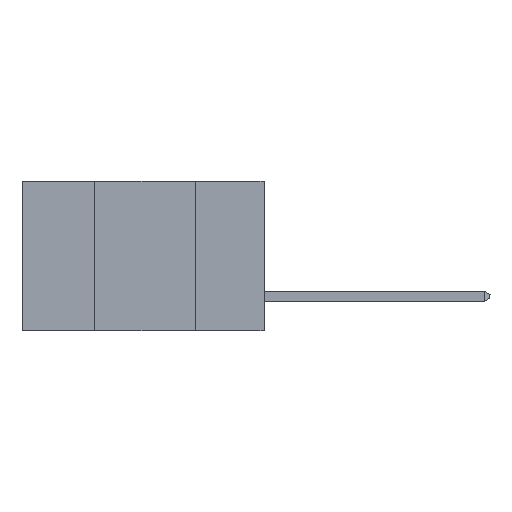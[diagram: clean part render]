
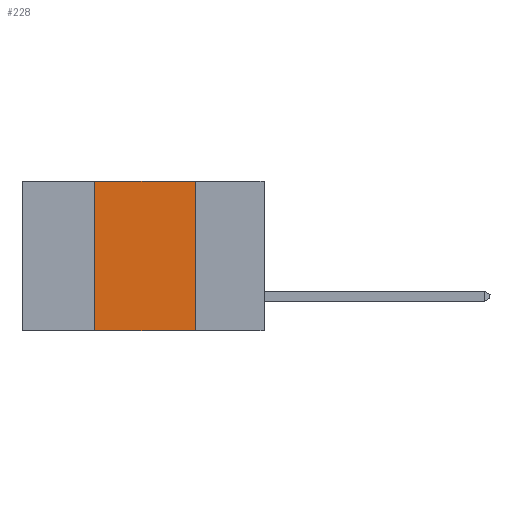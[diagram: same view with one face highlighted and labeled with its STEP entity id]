
A CAD part, left-side view. The second image highlights one B-rep face of the part: STEP entity #228.
In plain terms, the highlighted planar face has unit normal (-1, 0, 0).
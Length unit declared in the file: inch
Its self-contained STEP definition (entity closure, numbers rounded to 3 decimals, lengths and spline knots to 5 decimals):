
#207 = FACE_OUTER_BOUND ( 'NONE', #12482, .T. ) ;
#228 = ADVANCED_FACE ( 'NONE', ( #207 ), #3920, .F. ) ;
#1345 = LINE ( 'NONE', #12402, #24226 ) ;
#1505 = CARTESIAN_POINT ( 'NONE',  ( 0., 0.42, 0. ) ) ;
#3050 = VECTOR ( 'NONE', #22105, 39.37008 ) ;
#3715 = ORIENTED_EDGE ( 'NONE', *, *, #26645, .F. ) ;
#3920 = PLANE ( 'NONE',  #15016 ) ;
#5439 = LINE ( 'NONE', #12384, #25395 ) ;
#6491 = LINE ( 'NONE', #10390, #8286 ) ;
#8286 = VECTOR ( 'NONE', #26597, 39.37008 ) ;
#9565 = VERTEX_POINT ( 'NONE', #16654 ) ;
#10074 = DIRECTION ( 'NONE',  ( 0., 0., -1. ) ) ;
#10390 = CARTESIAN_POINT ( 'NONE',  ( 0., 0.6, -0.37 ) ) ;
#12120 = EDGE_CURVE ( 'NONE', #15894, #26851, #6491, .T. ) ;
#12350 = CARTESIAN_POINT ( 'NONE',  ( 0., 0.17, 0. ) ) ;
#12384 = CARTESIAN_POINT ( 'NONE',  ( 0., 0.6, 0. ) ) ;
#12402 = CARTESIAN_POINT ( 'NONE',  ( 0., 0.17, 0. ) ) ;
#12482 = EDGE_LOOP ( 'NONE', ( #26907, #29777, #3715, #27131 ) ) ;
#12529 = EDGE_CURVE ( 'NONE', #9565, #14720, #5439, .T. ) ;
#13251 = CARTESIAN_POINT ( 'NONE',  ( 0., 0.6, 0. ) ) ;
#13402 = CARTESIAN_POINT ( 'NONE',  ( 0., 0.17, -0.37 ) ) ;
#13560 = DIRECTION ( 'NONE',  ( 1., 0., 0. ) ) ;
#14720 = VERTEX_POINT ( 'NONE', #12350 ) ;
#14857 = CARTESIAN_POINT ( 'NONE',  ( 0., 0.42, -0.37 ) ) ;
#15016 = AXIS2_PLACEMENT_3D ( 'NONE', #13251, #13560, #18333 ) ;
#15894 = VERTEX_POINT ( 'NONE', #14857 ) ;
#16654 = CARTESIAN_POINT ( 'NONE',  ( 0., 0.42, 0. ) ) ;
#18333 = DIRECTION ( 'NONE',  ( 0., 0., -1. ) ) ;
#21580 = EDGE_CURVE ( 'NONE', #14720, #26851, #1345, .T. ) ;
#22105 = DIRECTION ( 'NONE',  ( 0., 0., 1. ) ) ;
#22639 = LINE ( 'NONE', #1505, #3050 ) ;
#24226 = VECTOR ( 'NONE', #10074, 39.37008 ) ;
#25395 = VECTOR ( 'NONE', #28622, 39.37008 ) ;
#26597 = DIRECTION ( 'NONE',  ( 0., -1., 0. ) ) ;
#26645 = EDGE_CURVE ( 'NONE', #15894, #9565, #22639, .T. ) ;
#26851 = VERTEX_POINT ( 'NONE', #13402 ) ;
#26907 = ORIENTED_EDGE ( 'NONE', *, *, #21580, .F. ) ;
#27131 = ORIENTED_EDGE ( 'NONE', *, *, #12120, .T. ) ;
#28622 = DIRECTION ( 'NONE',  ( 0., -1., 0. ) ) ;
#29777 = ORIENTED_EDGE ( 'NONE', *, *, #12529, .F. ) ;
